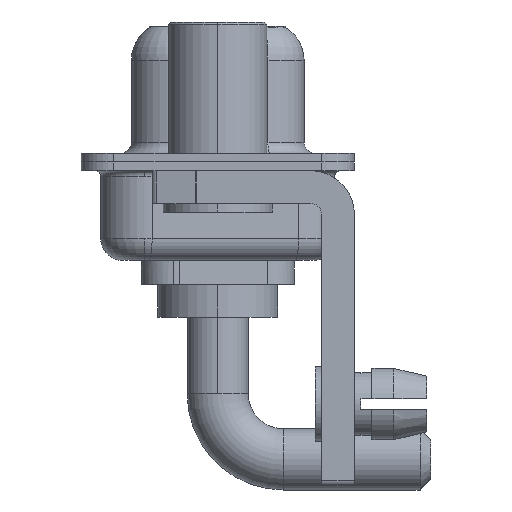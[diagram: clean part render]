
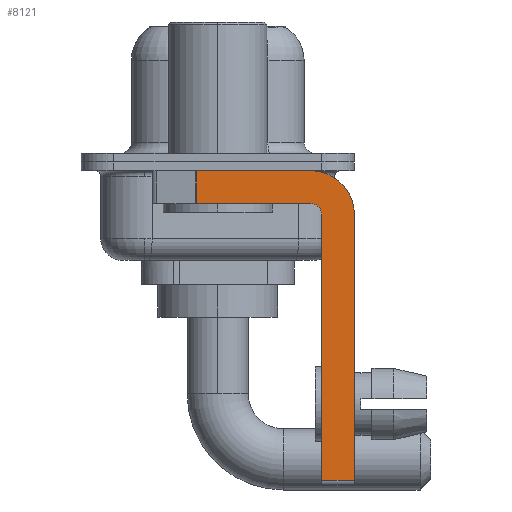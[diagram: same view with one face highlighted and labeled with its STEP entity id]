
A CAD part, left-side view. The second image highlights one B-rep face of the part: STEP entity #8121.
In plain terms, the highlighted planar face has unit normal (-1, 0, 0).
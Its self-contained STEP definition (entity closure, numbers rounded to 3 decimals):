
#32 = DIRECTION ( 'NONE',  ( 0., -1., 0. ) ) ;
#121 = EDGE_CURVE ( 'NONE', #308, #6087, #8828, .T. ) ;
#308 = VERTEX_POINT ( 'NONE', #1763 ) ;
#339 = LINE ( 'NONE', #12776, #10467 ) ;
#759 = EDGE_CURVE ( 'NONE', #9701, #4371, #339, .T. ) ;
#1281 = CARTESIAN_POINT ( 'NONE',  ( -2.9, 3., -0.4 ) ) ;
#1629 = VECTOR ( 'NONE', #7511, 1000. ) ;
#1763 = CARTESIAN_POINT ( 'NONE',  ( -2.9, -4.25, -1.9 ) ) ;
#1832 = CARTESIAN_POINT ( 'NONE',  ( -2.9, -6.25, -2.4 ) ) ;
#1868 = AXIS2_PLACEMENT_3D ( 'NONE', #14137, #8194, #15452 ) ;
#1972 = CARTESIAN_POINT ( 'NONE',  ( -2.9, 0.978, -1.9 ) ) ;
#2281 = AXIS2_PLACEMENT_3D ( 'NONE', #15644, #10470, #14414 ) ;
#2975 = VERTEX_POINT ( 'NONE', #1832 ) ;
#3020 = EDGE_CURVE ( 'NONE', #14444, #2975, #12275, .T. ) ;
#3682 = DIRECTION ( 'NONE',  ( 0., 0., 1. ) ) ;
#4032 = LINE ( 'NONE', #12601, #14714 ) ;
#4371 = VERTEX_POINT ( 'NONE', #16236 ) ;
#5153 = ORIENTED_EDGE ( 'NONE', *, *, #14667, .F. ) ;
#5218 = CARTESIAN_POINT ( 'NONE',  ( -2.9, -4.75, -2.4 ) ) ;
#6087 = VERTEX_POINT ( 'NONE', #1972 ) ;
#6818 = CARTESIAN_POINT ( 'NONE',  ( -2.9, -4.25, -0.4 ) ) ;
#7511 = DIRECTION ( 'NONE',  ( 0., 1., 0. ) ) ;
#7529 = EDGE_CURVE ( 'NONE', #14936, #6087, #8840, .T. ) ;
#7567 = CARTESIAN_POINT ( 'NONE',  ( -2.9, -4.25, -2.4 ) ) ;
#7761 = LINE ( 'NONE', #1281, #8198 ) ;
#8117 = ORIENTED_EDGE ( 'NONE', *, *, #7529, .T. ) ;
#8121 = ADVANCED_FACE ( 'NONE', ( #12517 ), #10213, .F. ) ;
#8144 = EDGE_CURVE ( 'NONE', #2975, #4371, #4032, .T. ) ;
#8194 = DIRECTION ( 'NONE',  ( -1., 0., 0. ) ) ;
#8198 = VECTOR ( 'NONE', #32, 1000. ) ;
#8666 = EDGE_CURVE ( 'NONE', #10516, #308, #9228, .T. ) ;
#8745 = CARTESIAN_POINT ( 'NONE',  ( -2.9, -4.25, -1.9 ) ) ;
#8763 = ORIENTED_EDGE ( 'NONE', *, *, #8144, .F. ) ;
#8828 = LINE ( 'NONE', #8745, #1629 ) ;
#8840 = LINE ( 'NONE', #10166, #11548 ) ;
#9214 = AXIS2_PLACEMENT_3D ( 'NONE', #7567, #12810, #15056 ) ;
#9228 = CIRCLE ( 'NONE', #1868, 0.5 ) ;
#9352 = CARTESIAN_POINT ( 'NONE',  ( -2.9, 0.978, -0.4 ) ) ;
#9701 = VERTEX_POINT ( 'NONE', #10797 ) ;
#10025 = ORIENTED_EDGE ( 'NONE', *, *, #8666, .F. ) ;
#10128 = DIRECTION ( 'NONE',  ( 0., 0., -1. ) ) ;
#10166 = CARTESIAN_POINT ( 'NONE',  ( -2.9, 0.978, -1.9 ) ) ;
#10213 = PLANE ( 'NONE',  #9214 ) ;
#10467 = VECTOR ( 'NONE', #14166, 1000. ) ;
#10470 = DIRECTION ( 'NONE',  ( 1., 0., 0. ) ) ;
#10516 = VERTEX_POINT ( 'NONE', #5218 ) ;
#10797 = CARTESIAN_POINT ( 'NONE',  ( -2.9, -4.75, -14.55 ) ) ;
#11007 = ORIENTED_EDGE ( 'NONE', *, *, #121, .F. ) ;
#11548 = VECTOR ( 'NONE', #16155, 1000. ) ;
#12084 = EDGE_CURVE ( 'NONE', #14936, #14444, #7761, .T. ) ;
#12275 = CIRCLE ( 'NONE', #2281, 2. ) ;
#12517 = FACE_OUTER_BOUND ( 'NONE', #14301, .T. ) ;
#12601 = CARTESIAN_POINT ( 'NONE',  ( -2.9, -6.25, -2.4 ) ) ;
#12744 = LINE ( 'NONE', #16258, #14046 ) ;
#12776 = CARTESIAN_POINT ( 'NONE',  ( -2.9, -4.25, -14.55 ) ) ;
#12810 = DIRECTION ( 'NONE',  ( 1., 0., 0. ) ) ;
#13215 = ORIENTED_EDGE ( 'NONE', *, *, #759, .T. ) ;
#14046 = VECTOR ( 'NONE', #3682, 1000. ) ;
#14137 = CARTESIAN_POINT ( 'NONE',  ( -2.9, -4.25, -2.4 ) ) ;
#14166 = DIRECTION ( 'NONE',  ( 0., -1., 0. ) ) ;
#14301 = EDGE_LOOP ( 'NONE', ( #15479, #8117, #11007, #10025, #5153, #13215, #8763, #16188 ) ) ;
#14414 = DIRECTION ( 'NONE',  ( 0., 0., -1. ) ) ;
#14444 = VERTEX_POINT ( 'NONE', #6818 ) ;
#14667 = EDGE_CURVE ( 'NONE', #9701, #10516, #12744, .T. ) ;
#14714 = VECTOR ( 'NONE', #10128, 1000. ) ;
#14936 = VERTEX_POINT ( 'NONE', #9352 ) ;
#15056 = DIRECTION ( 'NONE',  ( 0., 0., -1. ) ) ;
#15452 = DIRECTION ( 'NONE',  ( 0., 0., 1. ) ) ;
#15479 = ORIENTED_EDGE ( 'NONE', *, *, #12084, .F. ) ;
#15644 = CARTESIAN_POINT ( 'NONE',  ( -2.9, -4.25, -2.4 ) ) ;
#16155 = DIRECTION ( 'NONE',  ( 0., 0., -1. ) ) ;
#16188 = ORIENTED_EDGE ( 'NONE', *, *, #3020, .F. ) ;
#16236 = CARTESIAN_POINT ( 'NONE',  ( -2.9, -6.25, -14.55 ) ) ;
#16258 = CARTESIAN_POINT ( 'NONE',  ( -2.9, -4.75, -14.8 ) ) ;
